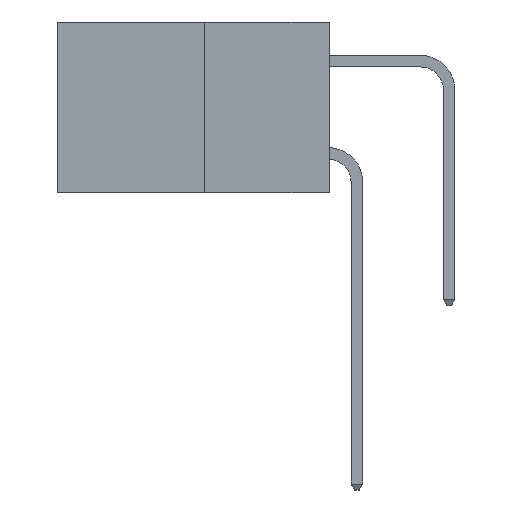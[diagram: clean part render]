
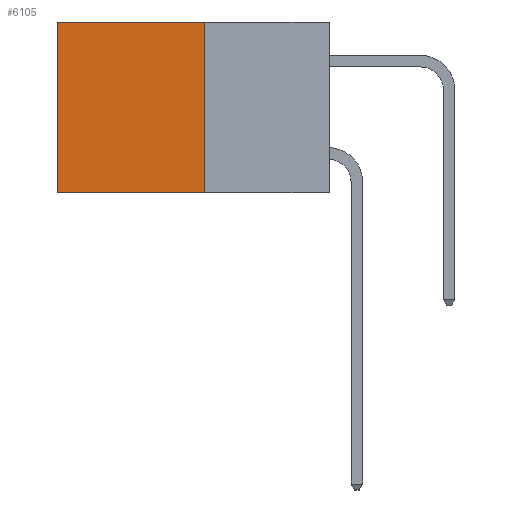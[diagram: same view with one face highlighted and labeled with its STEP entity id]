
A CAD part, left-side view. The second image highlights one B-rep face of the part: STEP entity #6105.
In plain terms, the highlighted planar face has unit normal (-1, 0, 0).
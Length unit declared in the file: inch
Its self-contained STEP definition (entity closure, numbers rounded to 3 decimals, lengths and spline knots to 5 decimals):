
#166 = CARTESIAN_POINT ( 'NONE',  ( 0.277, 0.59, -0.37 ) ) ;
#255 = DIRECTION ( 'NONE',  ( 0., 0., -1. ) ) ;
#841 = VERTEX_POINT ( 'NONE', #11170 ) ;
#1587 = DIRECTION ( 'NONE',  ( 0., 0., -1. ) ) ;
#1728 = CARTESIAN_POINT ( 'NONE',  ( 0.277, 0.59, -0.37 ) ) ;
#1968 = AXIS2_PLACEMENT_3D ( 'NONE', #5985, #7056, #255 ) ;
#2237 = VERTEX_POINT ( 'NONE', #166 ) ;
#2783 = CARTESIAN_POINT ( 'NONE',  ( 0.277, 0.27, -0.37 ) ) ;
#2888 = ORIENTED_EDGE ( 'NONE', *, *, #7341, .F. ) ;
#2918 = DIRECTION ( 'NONE',  ( 0., 0., -1. ) ) ;
#4337 = LINE ( 'NONE', #1728, #9807 ) ;
#4551 = EDGE_CURVE ( 'NONE', #7637, #8725, #6773, .T. ) ;
#4866 = PLANE ( 'NONE',  #1968 ) ;
#4881 = CARTESIAN_POINT ( 'NONE',  ( 0.277, 0.27, -0.37 ) ) ;
#4997 = CARTESIAN_POINT ( 'NONE',  ( 0.277, 0.59, 0. ) ) ;
#5876 = LINE ( 'NONE', #4881, #10784 ) ;
#5985 = CARTESIAN_POINT ( 'NONE',  ( 0.277, 0.27, -0.37 ) ) ;
#6002 = DIRECTION ( 'NONE',  ( 0., 1., 0. ) ) ;
#6105 = ADVANCED_FACE ( 'NONE', ( #6446 ), #4866, .F. ) ;
#6446 = FACE_OUTER_BOUND ( 'NONE', #10701, .T. ) ;
#6773 = LINE ( 'NONE', #10155, #11597 ) ;
#6988 = EDGE_CURVE ( 'NONE', #8725, #2237, #4337, .T. ) ;
#7056 = DIRECTION ( 'NONE',  ( 1., 0., 0. ) ) ;
#7341 = EDGE_CURVE ( 'NONE', #841, #2237, #5876, .T. ) ;
#7361 = VECTOR ( 'NONE', #1587, 39.37008 ) ;
#7510 = ORIENTED_EDGE ( 'NONE', *, *, #7895, .F. ) ;
#7513 = ORIENTED_EDGE ( 'NONE', *, *, #4551, .T. ) ;
#7637 = VERTEX_POINT ( 'NONE', #7770 ) ;
#7694 = LINE ( 'NONE', #2783, #7361 ) ;
#7770 = CARTESIAN_POINT ( 'NONE',  ( 0.277, 0.27, 0. ) ) ;
#7895 = EDGE_CURVE ( 'NONE', #7637, #841, #7694, .T. ) ;
#8725 = VERTEX_POINT ( 'NONE', #4997 ) ;
#9807 = VECTOR ( 'NONE', #2918, 39.37008 ) ;
#10155 = CARTESIAN_POINT ( 'NONE',  ( 0.277, 0.27, 0. ) ) ;
#10701 = EDGE_LOOP ( 'NONE', ( #13352, #2888, #7510, #7513 ) ) ;
#10784 = VECTOR ( 'NONE', #6002, 39.37008 ) ;
#11064 = DIRECTION ( 'NONE',  ( 0., 1., 0. ) ) ;
#11170 = CARTESIAN_POINT ( 'NONE',  ( 0.277, 0.27, -0.37 ) ) ;
#11597 = VECTOR ( 'NONE', #11064, 39.37008 ) ;
#13352 = ORIENTED_EDGE ( 'NONE', *, *, #6988, .T. ) ;
